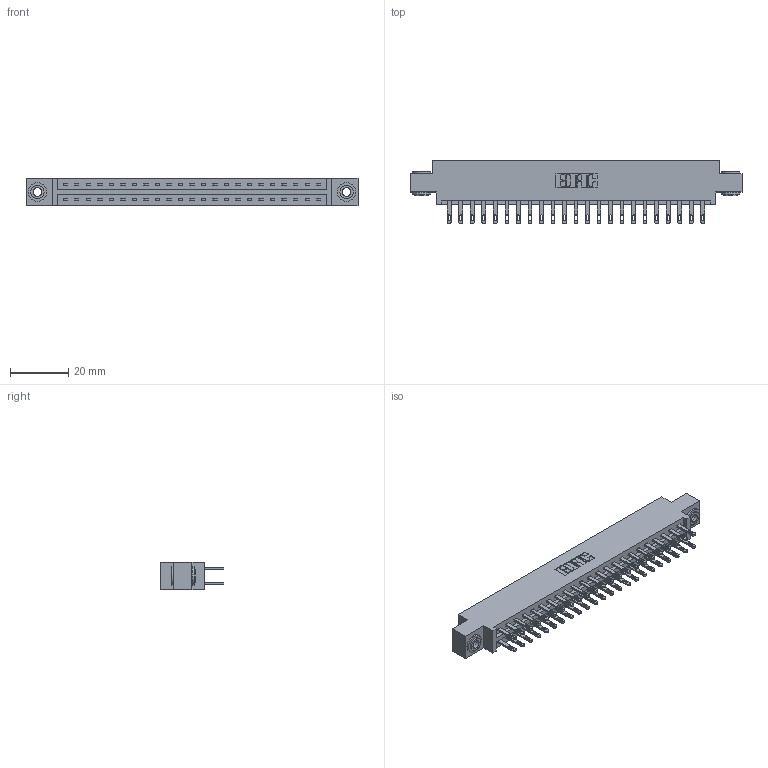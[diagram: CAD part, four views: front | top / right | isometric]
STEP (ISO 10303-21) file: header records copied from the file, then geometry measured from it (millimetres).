
FILE_DESCRIPTION (( 'STEP AP203' ), '1' );
FILE_NAME ('887-046-500-803.STEP', '2020-09-21T00:44:54', ( '' ), ( '' ), 'SwSTEP 2.0', 'SolidWorks 2020', '' );
FILE_SCHEMA (( 'CONFIG_CONTROL_DESIGN' ));
Length unit declared in the file: inch
Products named in the file (4): 887-046-500-803; 345-292-001_345-293-100; 837 Part_0.170 Offset - 0.156 Dia-TH; 345-250-002_345-250-002-102
Assembly tree (49 placements, depth 2):
  887-046-500-803
    837 Part_0.170 Offset - 0.156 Dia-TH
    345-292-001_345-293-100  x46
    345-250-002_345-250-002-102  x2
Bounding box: 114.15 x 21.85 x 9.4 mm (x, y, z)
Volume: 11819.3 mm3; surface area: 14019.9 mm2
Topology: 49 solids, 49 shells, 2456 faces, 7437 edges, 4954 vertices
Faces by surface type: plane 1556, cylinder 892, cone 8
Entity records: 21002 total; most frequent: CARTESIAN_POINT 3529, ORIENTED_EDGE 3458, DIRECTION 3071, EDGE_CURVE 1729, VECTOR 1573, LINE 1573, VERTEX_POINT 1150, AXIS2_PLACEMENT_3D 749
